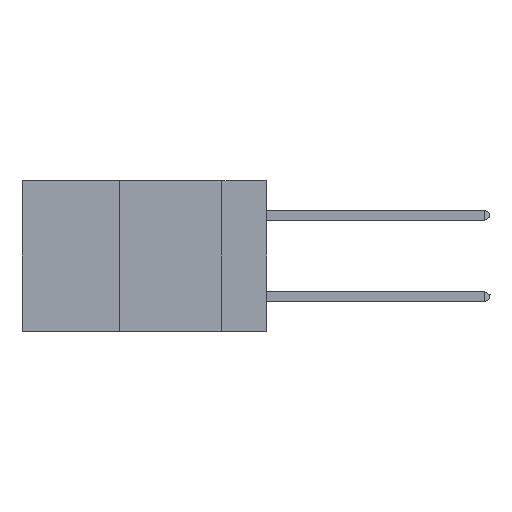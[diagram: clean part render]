
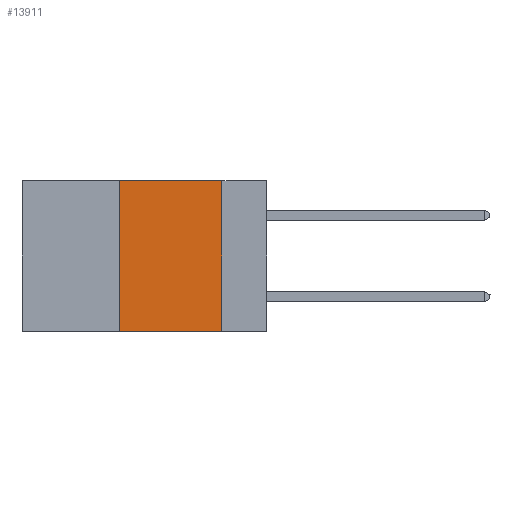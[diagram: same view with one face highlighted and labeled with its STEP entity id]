
A CAD part, left-side view. The second image highlights one B-rep face of the part: STEP entity #13911.
In plain terms, the highlighted planar face has unit normal (-1, 0, 0).
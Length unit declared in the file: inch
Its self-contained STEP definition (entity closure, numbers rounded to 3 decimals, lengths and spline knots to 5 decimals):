
#24 = LINE ( 'NONE', #12820, #9119 ) ;
#860 = ORIENTED_EDGE ( 'NONE', *, *, #1217, .F. ) ;
#1217 = EDGE_CURVE ( 'NONE', #5442, #12935, #3633, .T. ) ;
#1423 = DIRECTION ( 'NONE',  ( 0., -1., 0. ) ) ;
#1646 = CARTESIAN_POINT ( 'NONE',  ( 0., 0.36, 0. ) ) ;
#1789 = FACE_OUTER_BOUND ( 'NONE', #7430, .T. ) ;
#2393 = EDGE_CURVE ( 'NONE', #12935, #6162, #24, .T. ) ;
#2579 = VERTEX_POINT ( 'NONE', #2841 ) ;
#2712 = LINE ( 'NONE', #1646, #12035 ) ;
#2841 = CARTESIAN_POINT ( 'NONE',  ( 0., 0.36, -0.37 ) ) ;
#2863 = AXIS2_PLACEMENT_3D ( 'NONE', #13723, #6905, #5842 ) ;
#3633 = LINE ( 'NONE', #12373, #7355 ) ;
#5442 = VERTEX_POINT ( 'NONE', #10895 ) ;
#5842 = DIRECTION ( 'NONE',  ( 0., 0., -1. ) ) ;
#6162 = VERTEX_POINT ( 'NONE', #7226 ) ;
#6905 = DIRECTION ( 'NONE',  ( 1., 0., 0. ) ) ;
#7114 = PLANE ( 'NONE',  #2863 ) ;
#7148 = DIRECTION ( 'NONE',  ( 0., -1., 0. ) ) ;
#7226 = CARTESIAN_POINT ( 'NONE',  ( 0., 0.11, -0.37 ) ) ;
#7250 = DIRECTION ( 'NONE',  ( 0., 0., 1. ) ) ;
#7355 = VECTOR ( 'NONE', #1423, 39.37008 ) ;
#7430 = EDGE_LOOP ( 'NONE', ( #9392, #860, #7539, #7714 ) ) ;
#7539 = ORIENTED_EDGE ( 'NONE', *, *, #8370, .F. ) ;
#7714 = ORIENTED_EDGE ( 'NONE', *, *, #12821, .T. ) ;
#8370 = EDGE_CURVE ( 'NONE', #2579, #5442, #2712, .T. ) ;
#8586 = VECTOR ( 'NONE', #7148, 39.37008 ) ;
#9119 = VECTOR ( 'NONE', #9647, 39.37008 ) ;
#9369 = LINE ( 'NONE', #10233, #8586 ) ;
#9392 = ORIENTED_EDGE ( 'NONE', *, *, #2393, .F. ) ;
#9647 = DIRECTION ( 'NONE',  ( 0., 0., -1. ) ) ;
#10233 = CARTESIAN_POINT ( 'NONE',  ( 0., 0.6, -0.37 ) ) ;
#10895 = CARTESIAN_POINT ( 'NONE',  ( 0., 0.36, 0. ) ) ;
#11843 = CARTESIAN_POINT ( 'NONE',  ( 0., 0.11, 0. ) ) ;
#12035 = VECTOR ( 'NONE', #7250, 39.37008 ) ;
#12373 = CARTESIAN_POINT ( 'NONE',  ( 0., 0.6, 0. ) ) ;
#12820 = CARTESIAN_POINT ( 'NONE',  ( 0., 0.11, 0. ) ) ;
#12821 = EDGE_CURVE ( 'NONE', #2579, #6162, #9369, .T. ) ;
#12935 = VERTEX_POINT ( 'NONE', #11843 ) ;
#13723 = CARTESIAN_POINT ( 'NONE',  ( 0., 0.6, 0. ) ) ;
#13911 = ADVANCED_FACE ( 'NONE', ( #1789 ), #7114, .F. ) ;
